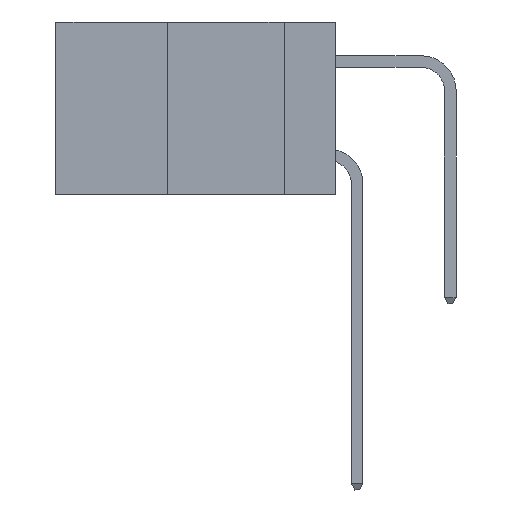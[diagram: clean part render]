
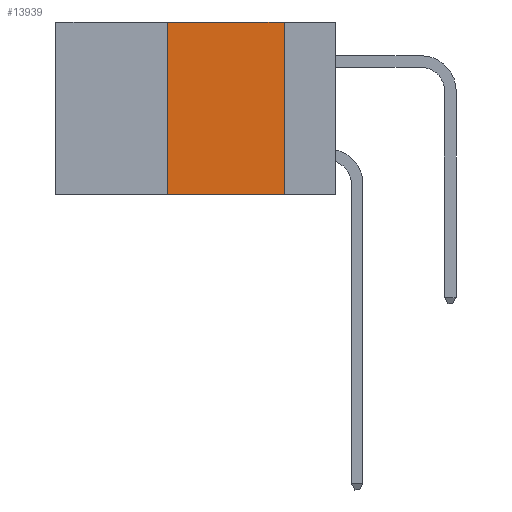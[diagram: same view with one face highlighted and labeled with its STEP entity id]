
A CAD part, left-side view. The second image highlights one B-rep face of the part: STEP entity #13939.
In plain terms, the highlighted planar face has unit normal (-1, 0, 0).
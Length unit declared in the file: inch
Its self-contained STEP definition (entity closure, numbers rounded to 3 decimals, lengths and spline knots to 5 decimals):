
#719 = VECTOR ( 'NONE', #8104, 39.37008 ) ;
#772 = VERTEX_POINT ( 'NONE', #4829 ) ;
#1077 = CARTESIAN_POINT ( 'NONE',  ( 0., 0.36, -0.37 ) ) ;
#1522 = DIRECTION ( 'NONE',  ( 0., 0., -1. ) ) ;
#1704 = CARTESIAN_POINT ( 'NONE',  ( 0., 0.11, -0.37 ) ) ;
#2012 = CARTESIAN_POINT ( 'NONE',  ( 0., 0.6, 0. ) ) ;
#3582 = DIRECTION ( 'NONE',  ( 0., 0., 1. ) ) ;
#4018 = LINE ( 'NONE', #7791, #7728 ) ;
#4274 = LINE ( 'NONE', #2012, #11244 ) ;
#4598 = LINE ( 'NONE', #5335, #719 ) ;
#4829 = CARTESIAN_POINT ( 'NONE',  ( 0., 0.36, 0. ) ) ;
#5127 = EDGE_CURVE ( 'NONE', #772, #6298, #4274, .T. ) ;
#5335 = CARTESIAN_POINT ( 'NONE',  ( 0., 0.11, 0. ) ) ;
#5402 = VECTOR ( 'NONE', #7974, 39.37008 ) ;
#6298 = VERTEX_POINT ( 'NONE', #11143 ) ;
#7728 = VECTOR ( 'NONE', #3582, 39.37008 ) ;
#7791 = CARTESIAN_POINT ( 'NONE',  ( 0., 0.36, 0. ) ) ;
#7974 = DIRECTION ( 'NONE',  ( 0., -1., 0. ) ) ;
#8104 = DIRECTION ( 'NONE',  ( 0., 0., -1. ) ) ;
#8539 = PLANE ( 'NONE',  #11954 ) ;
#9206 = FACE_OUTER_BOUND ( 'NONE', #15514, .T. ) ;
#9925 = DIRECTION ( 'NONE',  ( 1., 0., 0. ) ) ;
#11143 = CARTESIAN_POINT ( 'NONE',  ( 0., 0.11, 0. ) ) ;
#11244 = VECTOR ( 'NONE', #14641, 39.37008 ) ;
#11954 = AXIS2_PLACEMENT_3D ( 'NONE', #16946, #9925, #1522 ) ;
#12384 = LINE ( 'NONE', #16317, #5402 ) ;
#12941 = EDGE_CURVE ( 'NONE', #16624, #772, #4018, .T. ) ;
#13939 = ADVANCED_FACE ( 'NONE', ( #9206 ), #8539, .F. ) ;
#14638 = ORIENTED_EDGE ( 'NONE', *, *, #17765, .T. ) ;
#14641 = DIRECTION ( 'NONE',  ( 0., -1., 0. ) ) ;
#14670 = ORIENTED_EDGE ( 'NONE', *, *, #12941, .F. ) ;
#15263 = EDGE_CURVE ( 'NONE', #6298, #15573, #4598, .T. ) ;
#15514 = EDGE_LOOP ( 'NONE', ( #17063, #16977, #14670, #14638 ) ) ;
#15573 = VERTEX_POINT ( 'NONE', #1704 ) ;
#16317 = CARTESIAN_POINT ( 'NONE',  ( 0., 0.6, -0.37 ) ) ;
#16624 = VERTEX_POINT ( 'NONE', #1077 ) ;
#16946 = CARTESIAN_POINT ( 'NONE',  ( 0., 0.6, 0. ) ) ;
#16977 = ORIENTED_EDGE ( 'NONE', *, *, #5127, .F. ) ;
#17063 = ORIENTED_EDGE ( 'NONE', *, *, #15263, .F. ) ;
#17765 = EDGE_CURVE ( 'NONE', #16624, #15573, #12384, .T. ) ;
